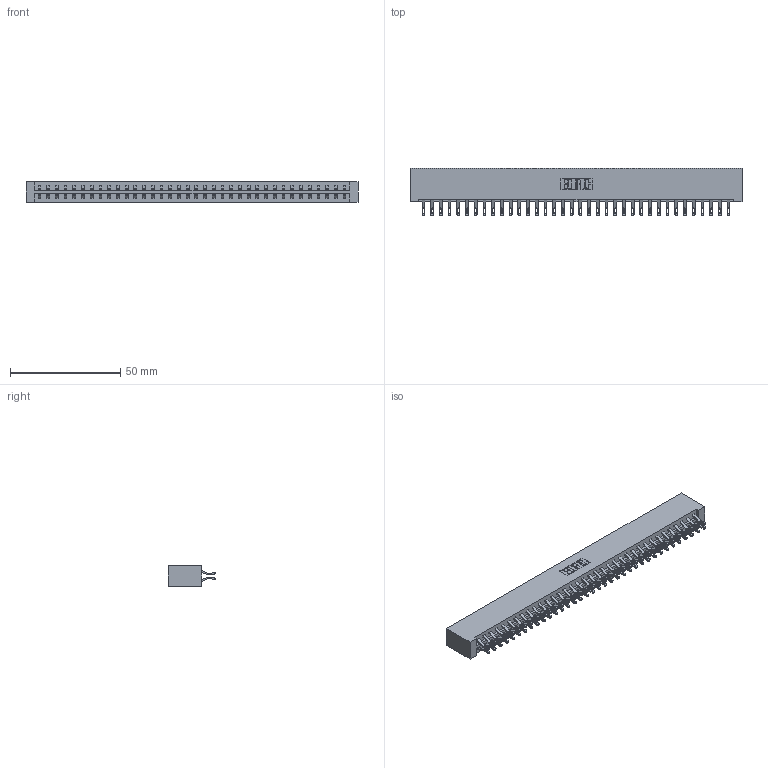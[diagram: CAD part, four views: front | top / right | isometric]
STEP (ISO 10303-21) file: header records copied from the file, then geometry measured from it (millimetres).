
FILE_DESCRIPTION (( 'STEP AP203' ), '1' );
FILE_NAME ('833-072-555-201.STEP', '2020-06-05T14:41:12', ( '' ), ( '' ), 'SwSTEP 2.0', 'SolidWorks 2020', '' );
FILE_SCHEMA (( 'CONFIG_CONTROL_DESIGN' ));
Length unit declared in the file: inch
Products named in the file (3): 833 Part_Lugless; 345-292-001_555 Tail; 833-072-555-201
Assembly tree (73 placements, depth 2):
  833-072-555-201
    833 Part_Lugless
    345-292-001_555 Tail  x72
Bounding box: 150.9 x 21.47 x 9.4 mm (x, y, z)
Volume: 16191.1 mm3; surface area: 19882.8 mm2
Topology: 73 solids, 73 shells, 4282 faces, 13463 edges, 8974 vertices
Faces by surface type: plane 2514, cylinder 1768
Entity records: 23985 total; most frequent: CARTESIAN_POINT 4016, ORIENTED_EDGE 3922, DIRECTION 3405, EDGE_CURVE 1961, LINE 1821, VECTOR 1821, VERTEX_POINT 1306, AXIS2_PLACEMENT_3D 792
